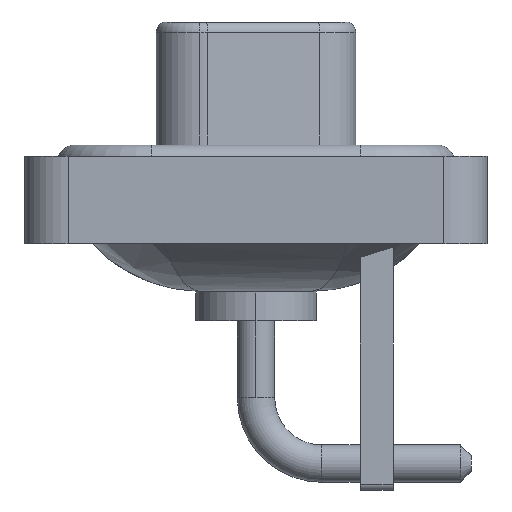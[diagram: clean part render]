
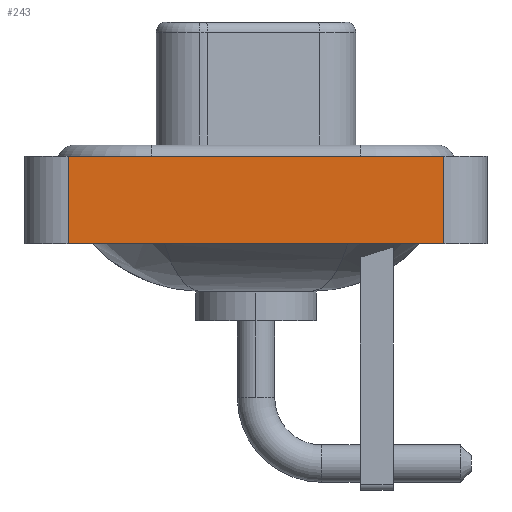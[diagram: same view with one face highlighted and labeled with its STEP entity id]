
A CAD part, left-side view. The second image highlights one B-rep face of the part: STEP entity #243.
In plain terms, the highlighted planar face has unit normal (-1, 0, 0).
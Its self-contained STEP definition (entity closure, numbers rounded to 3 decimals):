
#209 = CARTESIAN_POINT ( 'NONE',  ( -7.25, -8.55, 0.4 ) ) ;
#243 = ADVANCED_FACE ( 'NONE', ( #6985 ), #11886, .T. ) ;
#557 = LINE ( 'NONE', #15305, #10109 ) ;
#582 = ORIENTED_EDGE ( 'NONE', *, *, #12902, .T. ) ;
#904 = CARTESIAN_POINT ( 'NONE',  ( -7.25, -8.55, -3.6 ) ) ;
#1300 = DIRECTION ( 'NONE',  ( 0., 0., 1. ) ) ;
#1979 = EDGE_CURVE ( 'NONE', #6256, #14905, #5918, .T. ) ;
#2896 = CARTESIAN_POINT ( 'NONE',  ( -7.25, -8.55, -3.6 ) ) ;
#2950 = EDGE_CURVE ( 'NONE', #12984, #6256, #557, .T. ) ;
#3158 = DIRECTION ( 'NONE',  ( -1., 0., 0. ) ) ;
#4719 = CARTESIAN_POINT ( 'NONE',  ( -7.25, -8.55, -3.6 ) ) ;
#5012 = CARTESIAN_POINT ( 'NONE',  ( -7.25, 8.55, 0.4 ) ) ;
#5128 = EDGE_LOOP ( 'NONE', ( #582, #7723, #10780, #5633 ) ) ;
#5633 = ORIENTED_EDGE ( 'NONE', *, *, #12515, .T. ) ;
#5775 = DIRECTION ( 'NONE',  ( 0., 0., 1. ) ) ;
#5918 = LINE ( 'NONE', #9379, #14950 ) ;
#6256 = VERTEX_POINT ( 'NONE', #5012 ) ;
#6414 = LINE ( 'NONE', #2896, #9206 ) ;
#6486 = DIRECTION ( 'NONE',  ( 0., -1., 0. ) ) ;
#6985 = FACE_OUTER_BOUND ( 'NONE', #5128, .T. ) ;
#7367 = LINE ( 'NONE', #10827, #10252 ) ;
#7473 = VERTEX_POINT ( 'NONE', #4719 ) ;
#7723 = ORIENTED_EDGE ( 'NONE', *, *, #1979, .F. ) ;
#9206 = VECTOR ( 'NONE', #6486, 1000. ) ;
#9379 = CARTESIAN_POINT ( 'NONE',  ( -7.25, -8.55, 0.4 ) ) ;
#10047 = AXIS2_PLACEMENT_3D ( 'NONE', #904, #3158, #5775 ) ;
#10109 = VECTOR ( 'NONE', #12994, 1000. ) ;
#10252 = VECTOR ( 'NONE', #1300, 1000. ) ;
#10758 = DIRECTION ( 'NONE',  ( 0., -1., 0. ) ) ;
#10780 = ORIENTED_EDGE ( 'NONE', *, *, #2950, .F. ) ;
#10827 = CARTESIAN_POINT ( 'NONE',  ( -7.25, -8.55, -3.6 ) ) ;
#11886 = PLANE ( 'NONE',  #10047 ) ;
#12515 = EDGE_CURVE ( 'NONE', #12984, #7473, #6414, .T. ) ;
#12902 = EDGE_CURVE ( 'NONE', #7473, #14905, #7367, .T. ) ;
#12984 = VERTEX_POINT ( 'NONE', #13927 ) ;
#12994 = DIRECTION ( 'NONE',  ( 0., 0., 1. ) ) ;
#13927 = CARTESIAN_POINT ( 'NONE',  ( -7.25, 8.55, -3.6 ) ) ;
#14905 = VERTEX_POINT ( 'NONE', #209 ) ;
#14950 = VECTOR ( 'NONE', #10758, 1000. ) ;
#15305 = CARTESIAN_POINT ( 'NONE',  ( -7.25, 8.55, -3.6 ) ) ;
